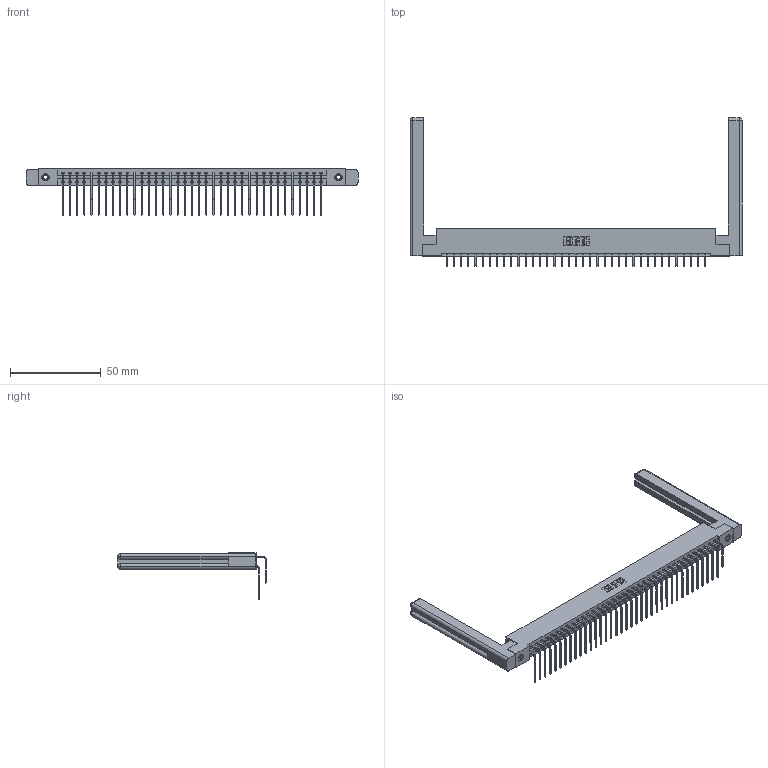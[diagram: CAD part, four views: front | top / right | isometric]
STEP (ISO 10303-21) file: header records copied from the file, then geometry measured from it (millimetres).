
FILE_DESCRIPTION (( 'STEP AP203' ), '1' );
FILE_NAME ('337-074-559-258.STEP', '2019-10-10T04:25:15', ( '' ), ( '' ), 'SwSTEP 2.0', 'SolidWorks 2016', '' );
FILE_SCHEMA (( 'CONFIG_CONTROL_DESIGN' ));
Length unit declared in the file: inch
Products named in the file (6): 337-074-559-258; 337 Part_Flush Mounting Lugs - 0.156 Dia-TI; 345-292-001_559 Tail - 2; 345-292-001_558 559 Tail - 1; 307-220-058; 345-250-001_345-250-001-102
Assembly tree (79 placements, depth 2):
  337-074-559-258
    337 Part_Flush Mounting Lugs - 0.156 Dia-TI
    345-292-001_558 559 Tail - 1  x37
    345-292-001_559 Tail - 2  x37
    345-250-001_345-250-001-102  x2
    307-220-058  x2
Bounding box: 183.24 x 81.98 x 25.53 mm (x, y, z)
Volume: 26813.5 mm3; surface area: 29380 mm2
Topology: 79 solids, 79 shells, 4400 faces, 13023 edges, 8570 vertices
Faces by surface type: plane 3114, cylinder 1262, cone 12, torus 12
Entity records: 33752 total; most frequent: CARTESIAN_POINT 5744, ORIENTED_EDGE 5568, DIRECTION 4892, EDGE_CURVE 2784, VECTOR 2568, LINE 2568, VERTEX_POINT 1846, AXIS2_PLACEMENT_3D 1162
